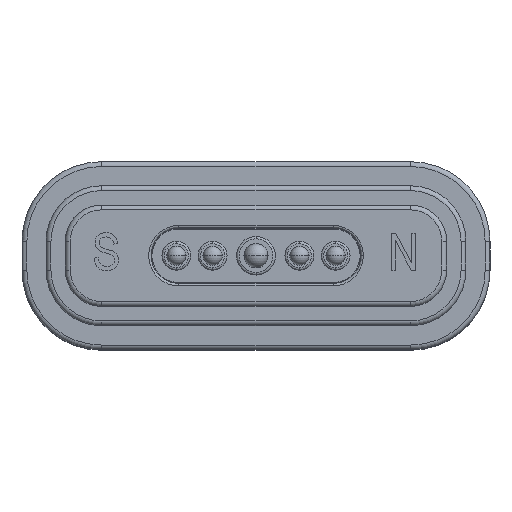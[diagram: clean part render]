
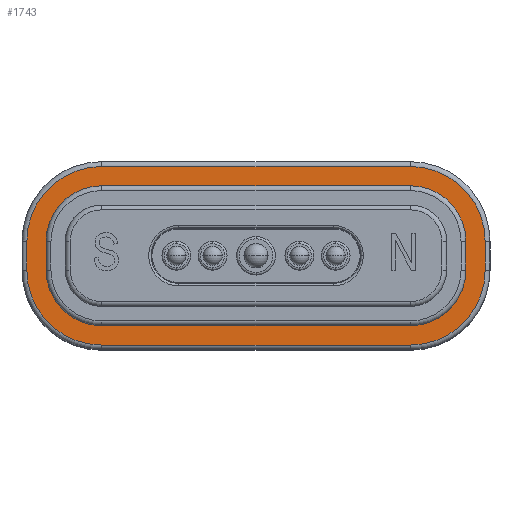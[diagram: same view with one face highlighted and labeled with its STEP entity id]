
A CAD part, top view. The second image highlights one B-rep face of the part: STEP entity #1743.
In plain terms, the highlighted planar face has unit normal (0, 0, 1).
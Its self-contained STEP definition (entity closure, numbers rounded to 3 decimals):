
#38 = DIRECTION ( 'NONE',  ( 0., -1., 0. ) ) ;
#158 = DIRECTION ( 'NONE',  ( 0., 0., -1. ) ) ;
#170 = EDGE_CURVE ( 'NONE', #7249, #1467, #7344, .T. ) ;
#176 = DIRECTION ( 'NONE',  ( 0., 0., -1. ) ) ;
#183 = AXIS2_PLACEMENT_3D ( 'NONE', #354, #158, #7141 ) ;
#271 = EDGE_LOOP ( 'NONE', ( #5506, #1940, #6872, #4593, #5382, #6967, #2633, #7539 ) ) ;
#354 = CARTESIAN_POINT ( 'NONE',  ( 6.4, 0.6, -0.79 ) ) ;
#390 = VERTEX_POINT ( 'NONE', #3443 ) ;
#464 = EDGE_CURVE ( 'NONE', #6488, #5315, #5423, .T. ) ;
#574 = CARTESIAN_POINT ( 'NONE',  ( -8.7, -0.6, -0.79 ) ) ;
#576 = CIRCLE ( 'NONE', #1123, 3.1 ) ;
#642 = EDGE_CURVE ( 'NONE', #1467, #3295, #7858, .T. ) ;
#734 = CIRCLE ( 'NONE', #183, 2.3 ) ;
#771 = VERTEX_POINT ( 'NONE', #3617 ) ;
#923 = DIRECTION ( 'NONE',  ( -1., 0., 0. ) ) ;
#930 = DIRECTION ( 'NONE',  ( 0., 0., 1. ) ) ;
#939 = CARTESIAN_POINT ( 'NONE',  ( -6.4, -0.6, -0.79 ) ) ;
#984 = VERTEX_POINT ( 'NONE', #1166 ) ;
#1001 = DIRECTION ( 'NONE',  ( 1., 0., 0. ) ) ;
#1115 = VECTOR ( 'NONE', #1001, 1000. ) ;
#1123 = AXIS2_PLACEMENT_3D ( 'NONE', #8186, #2467, #5026 ) ;
#1154 = AXIS2_PLACEMENT_3D ( 'NONE', #6174, #2593, #3176 ) ;
#1166 = CARTESIAN_POINT ( 'NONE',  ( 6.4, 2.9, -0.79 ) ) ;
#1395 = DIRECTION ( 'NONE',  ( 1., 0., 0. ) ) ;
#1409 = CIRCLE ( 'NONE', #4517, 3.1 ) ;
#1461 = CARTESIAN_POINT ( 'NONE',  ( -6.4, 3.7, -0.79 ) ) ;
#1467 = VERTEX_POINT ( 'NONE', #7117 ) ;
#1493 = VECTOR ( 'NONE', #4561, 1000. ) ;
#1612 = CARTESIAN_POINT ( 'NONE',  ( 6.4, -2.9, -0.79 ) ) ;
#1648 = CARTESIAN_POINT ( 'NONE',  ( 9.5, 0.6, -0.79 ) ) ;
#1667 = CARTESIAN_POINT ( 'NONE',  ( 6.4, -0.6, -0.79 ) ) ;
#1681 = CARTESIAN_POINT ( 'NONE',  ( 9.5, -0.6, -0.79 ) ) ;
#1743 = ADVANCED_FACE ( 'NONE', ( #3028, #4381 ), #8156, .T. ) ;
#1940 = ORIENTED_EDGE ( 'NONE', *, *, #2350, .T. ) ;
#1943 = AXIS2_PLACEMENT_3D ( 'NONE', #4183, #6396, #6422 ) ;
#2081 = CARTESIAN_POINT ( 'NONE',  ( 8.7, -0.6, -0.79 ) ) ;
#2090 = CARTESIAN_POINT ( 'NONE',  ( -9.5, 0.6, -0.79 ) ) ;
#2161 = EDGE_CURVE ( 'NONE', #5445, #3304, #1409, .T. ) ;
#2205 = CIRCLE ( 'NONE', #7005, 2.3 ) ;
#2229 = CARTESIAN_POINT ( 'NONE',  ( -6.4, 2.9, -0.79 ) ) ;
#2324 = DIRECTION ( 'NONE',  ( 0., 0., 1. ) ) ;
#2350 = EDGE_CURVE ( 'NONE', #7361, #5445, #3024, .T. ) ;
#2366 = CARTESIAN_POINT ( 'NONE',  ( -9.5, -0.6, -0.79 ) ) ;
#2467 = DIRECTION ( 'NONE',  ( 0., 0., 1. ) ) ;
#2593 = DIRECTION ( 'NONE',  ( 0., 0., -1. ) ) ;
#2633 = ORIENTED_EDGE ( 'NONE', *, *, #5220, .T. ) ;
#2878 = EDGE_CURVE ( 'NONE', #984, #6523, #734, .T. ) ;
#2907 = CIRCLE ( 'NONE', #1154, 2.3 ) ;
#2921 = ORIENTED_EDGE ( 'NONE', *, *, #5891, .T. ) ;
#2922 = VECTOR ( 'NONE', #6536, 1000. ) ;
#3022 = CIRCLE ( 'NONE', #1943, 3.1 ) ;
#3024 = LINE ( 'NONE', #2090, #1493 ) ;
#3028 = FACE_BOUND ( 'NONE', #5057, .T. ) ;
#3072 = EDGE_CURVE ( 'NONE', #6523, #6234, #8171, .T. ) ;
#3176 = DIRECTION ( 'NONE',  ( 0., -1., 0. ) ) ;
#3295 = VERTEX_POINT ( 'NONE', #2229 ) ;
#3304 = VERTEX_POINT ( 'NONE', #4528 ) ;
#3384 = DIRECTION ( 'NONE',  ( 0., 0., 1. ) ) ;
#3391 = ORIENTED_EDGE ( 'NONE', *, *, #642, .T. ) ;
#3409 = EDGE_CURVE ( 'NONE', #4704, #7249, #2907, .T. ) ;
#3420 = CARTESIAN_POINT ( 'NONE',  ( 6.4, 3.7, -0.79 ) ) ;
#3427 = DIRECTION ( 'NONE',  ( -1., 0., 0. ) ) ;
#3443 = CARTESIAN_POINT ( 'NONE',  ( 6.4, -3.7, -0.79 ) ) ;
#3509 = EDGE_CURVE ( 'NONE', #3295, #984, #7542, .T. ) ;
#3617 = CARTESIAN_POINT ( 'NONE',  ( 6.4, 3.7, -0.79 ) ) ;
#3629 = EDGE_CURVE ( 'NONE', #771, #6954, #7746, .T. ) ;
#4056 = CARTESIAN_POINT ( 'NONE',  ( 8.7, 0.6, -0.79 ) ) ;
#4183 = CARTESIAN_POINT ( 'NONE',  ( -6.4, 0.6, -0.79 ) ) ;
#4218 = LINE ( 'NONE', #6741, #1115 ) ;
#4246 = DIRECTION ( 'NONE',  ( 0., 0., -1. ) ) ;
#4284 = DIRECTION ( 'NONE',  ( 1., 0., 0. ) ) ;
#4366 = AXIS2_PLACEMENT_3D ( 'NONE', #6034, #3384, #8276 ) ;
#4381 = FACE_OUTER_BOUND ( 'NONE', #271, .T. ) ;
#4517 = AXIS2_PLACEMENT_3D ( 'NONE', #939, #930, #923 ) ;
#4524 = ORIENTED_EDGE ( 'NONE', *, *, #4994, .T. ) ;
#4525 = DIRECTION ( 'NONE',  ( 0., 1., 0. ) ) ;
#4528 = CARTESIAN_POINT ( 'NONE',  ( -6.4, -3.7, -0.79 ) ) ;
#4561 = DIRECTION ( 'NONE',  ( 0., -1., 0. ) ) ;
#4593 = ORIENTED_EDGE ( 'NONE', *, *, #7054, .T. ) ;
#4621 = CIRCLE ( 'NONE', #4366, 3.1 ) ;
#4704 = VERTEX_POINT ( 'NONE', #6516 ) ;
#4788 = EDGE_CURVE ( 'NONE', #6954, #7361, #3022, .T. ) ;
#4843 = LINE ( 'NONE', #6929, #6615 ) ;
#4994 = EDGE_CURVE ( 'NONE', #5567, #4704, #4843, .T. ) ;
#5026 = DIRECTION ( 'NONE',  ( 0., -1., 0. ) ) ;
#5057 = EDGE_LOOP ( 'NONE', ( #6369, #2921, #4524, #6400, #6526, #3391, #5268, #7591 ) ) ;
#5220 = EDGE_CURVE ( 'NONE', #5315, #771, #4621, .T. ) ;
#5268 = ORIENTED_EDGE ( 'NONE', *, *, #3509, .T. ) ;
#5315 = VERTEX_POINT ( 'NONE', #1648 ) ;
#5382 = ORIENTED_EDGE ( 'NONE', *, *, #6033, .T. ) ;
#5423 = LINE ( 'NONE', #1681, #7234 ) ;
#5445 = VERTEX_POINT ( 'NONE', #2366 ) ;
#5486 = CARTESIAN_POINT ( 'NONE',  ( -6.4, 2.9, -0.79 ) ) ;
#5506 = ORIENTED_EDGE ( 'NONE', *, *, #4788, .T. ) ;
#5567 = VERTEX_POINT ( 'NONE', #1612 ) ;
#5891 = EDGE_CURVE ( 'NONE', #6234, #5567, #2205, .T. ) ;
#6033 = EDGE_CURVE ( 'NONE', #390, #6488, #576, .T. ) ;
#6034 = CARTESIAN_POINT ( 'NONE',  ( 6.4, 0.6, -0.79 ) ) ;
#6174 = CARTESIAN_POINT ( 'NONE',  ( -6.4, -0.6, -0.79 ) ) ;
#6234 = VERTEX_POINT ( 'NONE', #2081 ) ;
#6356 = DIRECTION ( 'NONE',  ( 0., 1., 0. ) ) ;
#6369 = ORIENTED_EDGE ( 'NONE', *, *, #3072, .T. ) ;
#6396 = DIRECTION ( 'NONE',  ( 0., 0., 1. ) ) ;
#6400 = ORIENTED_EDGE ( 'NONE', *, *, #3409, .T. ) ;
#6422 = DIRECTION ( 'NONE',  ( 0., 1., 0. ) ) ;
#6488 = VERTEX_POINT ( 'NONE', #7704 ) ;
#6516 = CARTESIAN_POINT ( 'NONE',  ( -6.4, -2.9, -0.79 ) ) ;
#6523 = VERTEX_POINT ( 'NONE', #7823 ) ;
#6526 = ORIENTED_EDGE ( 'NONE', *, *, #170, .T. ) ;
#6536 = DIRECTION ( 'NONE',  ( -1., 0., 0. ) ) ;
#6615 = VECTOR ( 'NONE', #3427, 1000. ) ;
#6741 = CARTESIAN_POINT ( 'NONE',  ( -6.4, -3.7, -0.79 ) ) ;
#6769 = DIRECTION ( 'NONE',  ( 1., 0., 0. ) ) ;
#6872 = ORIENTED_EDGE ( 'NONE', *, *, #2161, .T. ) ;
#6929 = CARTESIAN_POINT ( 'NONE',  ( 6.4, -2.9, -0.79 ) ) ;
#6954 = VERTEX_POINT ( 'NONE', #1461 ) ;
#6967 = ORIENTED_EDGE ( 'NONE', *, *, #464, .T. ) ;
#6979 = CARTESIAN_POINT ( 'NONE',  ( -6.4, 0.6, -0.79 ) ) ;
#7005 = AXIS2_PLACEMENT_3D ( 'NONE', #1667, #4246, #6769 ) ;
#7048 = CARTESIAN_POINT ( 'NONE',  ( -8.7, -0.6, -0.79 ) ) ;
#7054 = EDGE_CURVE ( 'NONE', #3304, #390, #4218, .T. ) ;
#7099 = AXIS2_PLACEMENT_3D ( 'NONE', #7405, #2324, #4284 ) ;
#7117 = CARTESIAN_POINT ( 'NONE',  ( -8.7, 0.6, -0.79 ) ) ;
#7141 = DIRECTION ( 'NONE',  ( 0., 1., 0. ) ) ;
#7189 = CARTESIAN_POINT ( 'NONE',  ( -9.5, 0.6, -0.79 ) ) ;
#7191 = VECTOR ( 'NONE', #1395, 1000. ) ;
#7234 = VECTOR ( 'NONE', #6356, 1000. ) ;
#7249 = VERTEX_POINT ( 'NONE', #574 ) ;
#7284 = DIRECTION ( 'NONE',  ( -1., 0., 0. ) ) ;
#7344 = LINE ( 'NONE', #7048, #8298 ) ;
#7348 = AXIS2_PLACEMENT_3D ( 'NONE', #6979, #176, #7284 ) ;
#7361 = VERTEX_POINT ( 'NONE', #7189 ) ;
#7405 = CARTESIAN_POINT ( 'NONE',  ( 0., 0., -0.79 ) ) ;
#7539 = ORIENTED_EDGE ( 'NONE', *, *, #3629, .T. ) ;
#7542 = LINE ( 'NONE', #5486, #7191 ) ;
#7581 = VECTOR ( 'NONE', #38, 1000. ) ;
#7591 = ORIENTED_EDGE ( 'NONE', *, *, #2878, .T. ) ;
#7704 = CARTESIAN_POINT ( 'NONE',  ( 9.5, -0.6, -0.79 ) ) ;
#7746 = LINE ( 'NONE', #3420, #2922 ) ;
#7823 = CARTESIAN_POINT ( 'NONE',  ( 8.7, 0.6, -0.79 ) ) ;
#7858 = CIRCLE ( 'NONE', #7348, 2.3 ) ;
#8156 = PLANE ( 'NONE',  #7099 ) ;
#8171 = LINE ( 'NONE', #4056, #7581 ) ;
#8186 = CARTESIAN_POINT ( 'NONE',  ( 6.4, -0.6, -0.79 ) ) ;
#8276 = DIRECTION ( 'NONE',  ( 1., 0., 0. ) ) ;
#8298 = VECTOR ( 'NONE', #4525, 1000. ) ;
